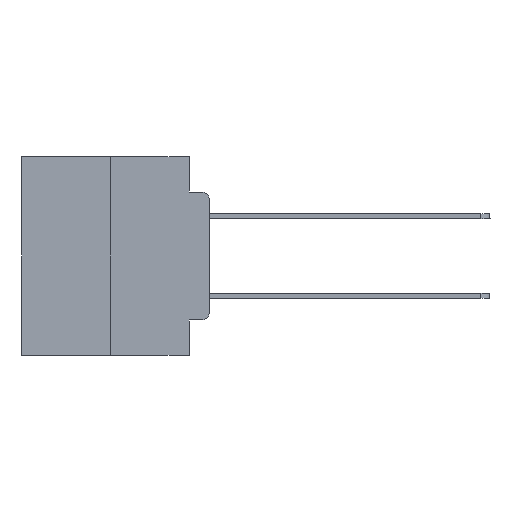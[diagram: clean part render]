
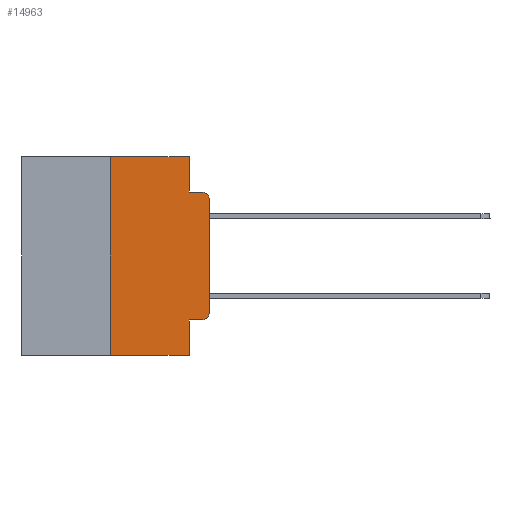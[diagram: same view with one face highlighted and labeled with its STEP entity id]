
A CAD part, left-side view. The second image highlights one B-rep face of the part: STEP entity #14963.
In plain terms, the highlighted planar face has unit normal (-1, 0, 0).
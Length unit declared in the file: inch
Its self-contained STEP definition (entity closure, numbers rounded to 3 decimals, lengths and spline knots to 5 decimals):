
#89 = DIRECTION ( 'NONE',  ( -1., 0., 0. ) ) ;
#91 = DIRECTION ( 'NONE',  ( 0., -1., 0. ) ) ;
#520 = DIRECTION ( 'NONE',  ( 0., -1., 0. ) ) ;
#1027 = VECTOR ( 'NONE', #26587, 39.37008 ) ;
#1949 = DIRECTION ( 'NONE',  ( 0., 0., 1. ) ) ;
#1968 = EDGE_CURVE ( 'NONE', #11073, #15184, #5330, .T. ) ;
#2039 = CARTESIAN_POINT ( 'NONE',  ( 0., 0., -0.3915 ) ) ;
#2047 = CARTESIAN_POINT ( 'NONE',  ( 0., 0.25, 0. ) ) ;
#2120 = VERTEX_POINT ( 'NONE', #4851 ) ;
#2371 = VECTOR ( 'NONE', #8073, 39.37008 ) ;
#2663 = VERTEX_POINT ( 'NONE', #2039 ) ;
#2783 = VERTEX_POINT ( 'NONE', #4906 ) ;
#3521 = AXIS2_PLACEMENT_3D ( 'NONE', #27756, #89, #4214 ) ;
#4214 = DIRECTION ( 'NONE',  ( 0., 0., -1. ) ) ;
#4420 = ORIENTED_EDGE ( 'NONE', *, *, #1968, .T. ) ;
#4583 = CARTESIAN_POINT ( 'NONE',  ( 0., 0.25, 0. ) ) ;
#4851 = CARTESIAN_POINT ( 'NONE',  ( 0., 0.051, -0.4115 ) ) ;
#4906 = CARTESIAN_POINT ( 'NONE',  ( 0., 0.02, -0.4115 ) ) ;
#5135 = CIRCLE ( 'NONE', #9110, 0.02 ) ;
#5204 = ORIENTED_EDGE ( 'NONE', *, *, #7420, .F. ) ;
#5330 = CIRCLE ( 'NONE', #3521, 0.02 ) ;
#5409 = PLANE ( 'NONE',  #18606 ) ;
#6074 = ORIENTED_EDGE ( 'NONE', *, *, #23626, .T. ) ;
#6655 = VECTOR ( 'NONE', #91, 39.37008 ) ;
#7420 = EDGE_CURVE ( 'NONE', #9996, #15184, #14407, .T. ) ;
#7442 = ORIENTED_EDGE ( 'NONE', *, *, #9909, .F. ) ;
#7783 = DIRECTION ( 'NONE',  ( 0., -1., 0. ) ) ;
#8010 = ORIENTED_EDGE ( 'NONE', *, *, #21668, .T. ) ;
#8073 = DIRECTION ( 'NONE',  ( 0., -1., 0. ) ) ;
#8876 = CARTESIAN_POINT ( 'NONE',  ( 0., 0.051, -0.4115 ) ) ;
#9110 = AXIS2_PLACEMENT_3D ( 'NONE', #16327, #23055, #12099 ) ;
#9140 = EDGE_LOOP ( 'NONE', ( #6074, #4420, #5204, #20840, #9554, #24397, #8010, #7442, #24587, #19479 ) ) ;
#9150 = CARTESIAN_POINT ( 'NONE',  ( 0., 0.051, -0.0885 ) ) ;
#9344 = DIRECTION ( 'NONE',  ( 0., 0., -1. ) ) ;
#9554 = ORIENTED_EDGE ( 'NONE', *, *, #13536, .F. ) ;
#9785 = CARTESIAN_POINT ( 'NONE',  ( 0., 0., 0. ) ) ;
#9909 = EDGE_CURVE ( 'NONE', #2120, #10385, #14942, .T. ) ;
#9996 = VERTEX_POINT ( 'NONE', #9150 ) ;
#10309 = EDGE_CURVE ( 'NONE', #20791, #9996, #24734, .T. ) ;
#10385 = VERTEX_POINT ( 'NONE', #18522 ) ;
#11073 = VERTEX_POINT ( 'NONE', #21980 ) ;
#11678 = LINE ( 'NONE', #18481, #25154 ) ;
#12099 = DIRECTION ( 'NONE',  ( 0., 0., -1. ) ) ;
#12554 = CARTESIAN_POINT ( 'NONE',  ( 0., 0.051, -0.0885 ) ) ;
#12620 = VECTOR ( 'NONE', #25098, 39.37008 ) ;
#13205 = LINE ( 'NONE', #2047, #23933 ) ;
#13536 = EDGE_CURVE ( 'NONE', #24383, #20791, #25038, .T. ) ;
#13593 = VECTOR ( 'NONE', #520, 39.37008 ) ;
#14268 = VECTOR ( 'NONE', #14946, 39.37008 ) ;
#14407 = LINE ( 'NONE', #12554, #2371 ) ;
#14851 = CARTESIAN_POINT ( 'NONE',  ( 0., 0.051, 0. ) ) ;
#14942 = LINE ( 'NONE', #14851, #14268 ) ;
#14946 = DIRECTION ( 'NONE',  ( 0., 0., -1. ) ) ;
#14963 = ADVANCED_FACE ( 'NONE', ( #18714 ), #5409, .F. ) ;
#15184 = VERTEX_POINT ( 'NONE', #24629 ) ;
#15610 = CARTESIAN_POINT ( 'NONE',  ( 0., 0.25, -0.5 ) ) ;
#15891 = CARTESIAN_POINT ( 'NONE',  ( 0., 0.473, 0. ) ) ;
#16085 = DIRECTION ( 'NONE',  ( 1., 0., 0. ) ) ;
#16327 = CARTESIAN_POINT ( 'NONE',  ( 0., 0.02, -0.3915 ) ) ;
#16954 = EDGE_CURVE ( 'NONE', #18150, #24383, #13205, .T. ) ;
#17074 = LINE ( 'NONE', #8876, #6655 ) ;
#17488 = EDGE_CURVE ( 'NONE', #2783, #2663, #5135, .T. ) ;
#18150 = VERTEX_POINT ( 'NONE', #15610 ) ;
#18481 = CARTESIAN_POINT ( 'NONE',  ( 0., 0.473, -0.5 ) ) ;
#18522 = CARTESIAN_POINT ( 'NONE',  ( 0., 0.051, -0.5 ) ) ;
#18606 = AXIS2_PLACEMENT_3D ( 'NONE', #15891, #16085, #9344 ) ;
#18714 = FACE_OUTER_BOUND ( 'NONE', #9140, .T. ) ;
#19479 = ORIENTED_EDGE ( 'NONE', *, *, #17488, .T. ) ;
#20448 = CARTESIAN_POINT ( 'NONE',  ( 0., 0.051, 0. ) ) ;
#20791 = VERTEX_POINT ( 'NONE', #20448 ) ;
#20840 = ORIENTED_EDGE ( 'NONE', *, *, #10309, .F. ) ;
#21668 = EDGE_CURVE ( 'NONE', #18150, #10385, #11678, .T. ) ;
#21980 = CARTESIAN_POINT ( 'NONE',  ( 0., 0., -0.1085 ) ) ;
#22004 = EDGE_CURVE ( 'NONE', #2120, #2783, #17074, .T. ) ;
#22713 = LINE ( 'NONE', #9785, #1027 ) ;
#23055 = DIRECTION ( 'NONE',  ( -1., 0., 0. ) ) ;
#23626 = EDGE_CURVE ( 'NONE', #2663, #11073, #22713, .T. ) ;
#23933 = VECTOR ( 'NONE', #1949, 39.37008 ) ;
#24383 = VERTEX_POINT ( 'NONE', #4583 ) ;
#24397 = ORIENTED_EDGE ( 'NONE', *, *, #16954, .F. ) ;
#24587 = ORIENTED_EDGE ( 'NONE', *, *, #22004, .T. ) ;
#24629 = CARTESIAN_POINT ( 'NONE',  ( 0., 0.02, -0.0885 ) ) ;
#24734 = LINE ( 'NONE', #27266, #12620 ) ;
#25038 = LINE ( 'NONE', #26589, #13593 ) ;
#25098 = DIRECTION ( 'NONE',  ( 0., 0., -1. ) ) ;
#25154 = VECTOR ( 'NONE', #7783, 39.37008 ) ;
#26587 = DIRECTION ( 'NONE',  ( 0., 0., 1. ) ) ;
#26589 = CARTESIAN_POINT ( 'NONE',  ( 0., 0.473, 0. ) ) ;
#27266 = CARTESIAN_POINT ( 'NONE',  ( 0., 0.051, 0. ) ) ;
#27756 = CARTESIAN_POINT ( 'NONE',  ( 0., 0.02, -0.1085 ) ) ;
